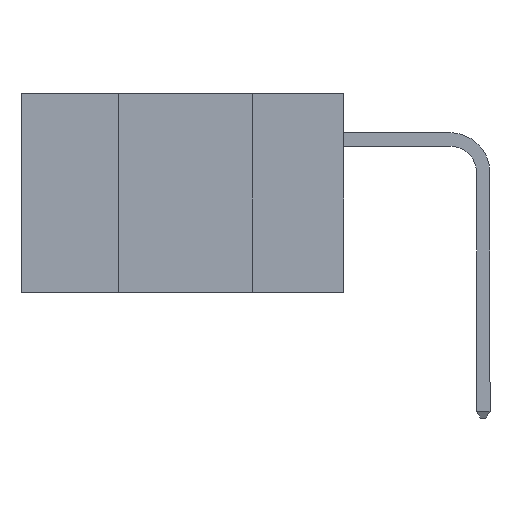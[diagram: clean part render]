
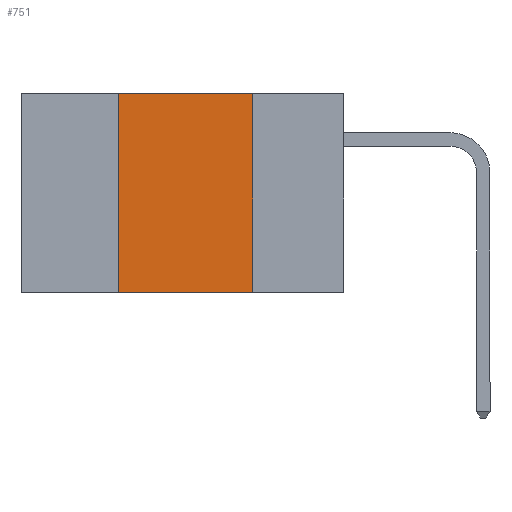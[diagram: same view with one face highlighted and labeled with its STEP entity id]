
A CAD part, left-side view. The second image highlights one B-rep face of the part: STEP entity #751.
In plain terms, the highlighted planar face has unit normal (-1, 0, 0).
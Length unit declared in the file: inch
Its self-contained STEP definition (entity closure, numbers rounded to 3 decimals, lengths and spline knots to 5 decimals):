
#174 = CARTESIAN_POINT ( 'NONE',  ( 0., 0.42, 0. ) ) ;
#595 = VECTOR ( 'NONE', #16676, 39.37008 ) ;
#751 = ADVANCED_FACE ( 'NONE', ( #9907 ), #15968, .F. ) ;
#1073 = LINE ( 'NONE', #18234, #595 ) ;
#1970 = ORIENTED_EDGE ( 'NONE', *, *, #3288, .T. ) ;
#2666 = VERTEX_POINT ( 'NONE', #13818 ) ;
#3047 = EDGE_CURVE ( 'NONE', #12411, #4439, #19535, .T. ) ;
#3288 = EDGE_CURVE ( 'NONE', #12411, #2666, #12138, .T. ) ;
#3519 = VECTOR ( 'NONE', #14361, 39.37008 ) ;
#3832 = CARTESIAN_POINT ( 'NONE',  ( 0., 0.42, 0. ) ) ;
#4101 = EDGE_CURVE ( 'NONE', #4439, #18202, #9515, .T. ) ;
#4439 = VERTEX_POINT ( 'NONE', #3832 ) ;
#4509 = DIRECTION ( 'NONE',  ( 0., -1., 0. ) ) ;
#5224 = EDGE_LOOP ( 'NONE', ( #11542, #19174, #14152, #1970 ) ) ;
#5544 = DIRECTION ( 'NONE',  ( 0., 0., -1. ) ) ;
#5559 = DIRECTION ( 'NONE',  ( 1., 0., 0. ) ) ;
#5581 = CARTESIAN_POINT ( 'NONE',  ( 0., 0.6, 0. ) ) ;
#9515 = LINE ( 'NONE', #14287, #16638 ) ;
#9595 = EDGE_CURVE ( 'NONE', #18202, #2666, #1073, .T. ) ;
#9624 = CARTESIAN_POINT ( 'NONE',  ( 0., 0.42, -0.37 ) ) ;
#9907 = FACE_OUTER_BOUND ( 'NONE', #5224, .T. ) ;
#10191 = AXIS2_PLACEMENT_3D ( 'NONE', #5581, #5559, #5544 ) ;
#11185 = DIRECTION ( 'NONE',  ( 0., 0., 1. ) ) ;
#11542 = ORIENTED_EDGE ( 'NONE', *, *, #9595, .F. ) ;
#12138 = LINE ( 'NONE', #16958, #3519 ) ;
#12411 = VERTEX_POINT ( 'NONE', #9624 ) ;
#13818 = CARTESIAN_POINT ( 'NONE',  ( 0., 0.17, -0.37 ) ) ;
#14152 = ORIENTED_EDGE ( 'NONE', *, *, #3047, .F. ) ;
#14287 = CARTESIAN_POINT ( 'NONE',  ( 0., 0.6, 0. ) ) ;
#14361 = DIRECTION ( 'NONE',  ( 0., -1., 0. ) ) ;
#15481 = VECTOR ( 'NONE', #11185, 39.37008 ) ;
#15925 = CARTESIAN_POINT ( 'NONE',  ( 0., 0.17, 0. ) ) ;
#15968 = PLANE ( 'NONE',  #10191 ) ;
#16638 = VECTOR ( 'NONE', #4509, 39.37008 ) ;
#16676 = DIRECTION ( 'NONE',  ( 0., 0., -1. ) ) ;
#16958 = CARTESIAN_POINT ( 'NONE',  ( 0., 0.6, -0.37 ) ) ;
#18202 = VERTEX_POINT ( 'NONE', #15925 ) ;
#18234 = CARTESIAN_POINT ( 'NONE',  ( 0., 0.17, 0. ) ) ;
#19174 = ORIENTED_EDGE ( 'NONE', *, *, #4101, .F. ) ;
#19535 = LINE ( 'NONE', #174, #15481 ) ;
